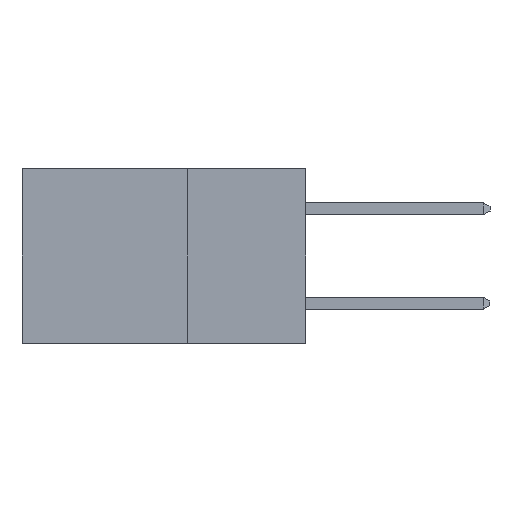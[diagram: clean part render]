
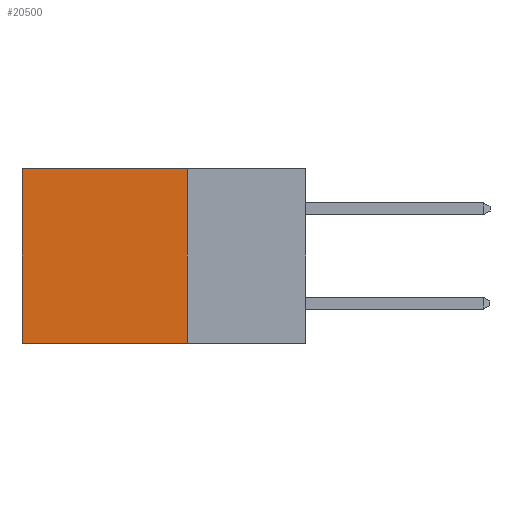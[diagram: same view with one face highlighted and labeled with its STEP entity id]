
A CAD part, left-side view. The second image highlights one B-rep face of the part: STEP entity #20500.
In plain terms, the highlighted planar face has unit normal (-1, 0, 0).
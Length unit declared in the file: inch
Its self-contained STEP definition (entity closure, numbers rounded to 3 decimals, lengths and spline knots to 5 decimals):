
#553 = FACE_OUTER_BOUND ( 'NONE', #14517, .T. ) ;
#619 = DIRECTION ( 'NONE',  ( 0., 0., -1. ) ) ;
#724 = VERTEX_POINT ( 'NONE', #21676 ) ;
#782 = CARTESIAN_POINT ( 'NONE',  ( 0.298, 0.6, 0. ) ) ;
#848 = PLANE ( 'NONE',  #11613 ) ;
#854 = ORIENTED_EDGE ( 'NONE', *, *, #21178, .F. ) ;
#1084 = CARTESIAN_POINT ( 'NONE',  ( 0.298, 0.25, 0. ) ) ;
#1229 = CARTESIAN_POINT ( 'NONE',  ( 0.298, 0.25, 0. ) ) ;
#1475 = LINE ( 'NONE', #15895, #19737 ) ;
#1815 = VERTEX_POINT ( 'NONE', #14395 ) ;
#2635 = DIRECTION ( 'NONE',  ( 0., 0., -1. ) ) ;
#3260 = ORIENTED_EDGE ( 'NONE', *, *, #22896, .T. ) ;
#3874 = LINE ( 'NONE', #1084, #17453 ) ;
#4594 = VERTEX_POINT ( 'NONE', #1229 ) ;
#4924 = ORIENTED_EDGE ( 'NONE', *, *, #20806, .T. ) ;
#6102 = CARTESIAN_POINT ( 'NONE',  ( 0.298, 0.25, 0. ) ) ;
#9103 = VECTOR ( 'NONE', #619, 39.37008 ) ;
#9323 = VERTEX_POINT ( 'NONE', #22578 ) ;
#9467 = CARTESIAN_POINT ( 'NONE',  ( 0.298, 0.25, 0. ) ) ;
#9681 = LINE ( 'NONE', #9467, #9103 ) ;
#11015 = LINE ( 'NONE', #782, #15130 ) ;
#11392 = DIRECTION ( 'NONE',  ( 0., 0., -1. ) ) ;
#11613 = AXIS2_PLACEMENT_3D ( 'NONE', #6102, #13232, #2635 ) ;
#11621 = DIRECTION ( 'NONE',  ( 0., 1., 0. ) ) ;
#12949 = ORIENTED_EDGE ( 'NONE', *, *, #18917, .F. ) ;
#13232 = DIRECTION ( 'NONE',  ( 1., 0., 0. ) ) ;
#14210 = DIRECTION ( 'NONE',  ( 0., 1., 0. ) ) ;
#14395 = CARTESIAN_POINT ( 'NONE',  ( 0.298, 0.6, 0. ) ) ;
#14517 = EDGE_LOOP ( 'NONE', ( #3260, #12949, #854, #4924 ) ) ;
#15130 = VECTOR ( 'NONE', #11392, 39.37008 ) ;
#15895 = CARTESIAN_POINT ( 'NONE',  ( 0.298, 0.25, -0.37 ) ) ;
#17453 = VECTOR ( 'NONE', #11621, 39.37008 ) ;
#18917 = EDGE_CURVE ( 'NONE', #9323, #724, #1475, .T. ) ;
#19737 = VECTOR ( 'NONE', #14210, 39.37008 ) ;
#20500 = ADVANCED_FACE ( 'NONE', ( #553 ), #848, .F. ) ;
#20806 = EDGE_CURVE ( 'NONE', #4594, #1815, #3874, .T. ) ;
#21178 = EDGE_CURVE ( 'NONE', #4594, #9323, #9681, .T. ) ;
#21676 = CARTESIAN_POINT ( 'NONE',  ( 0.298, 0.6, -0.37 ) ) ;
#22578 = CARTESIAN_POINT ( 'NONE',  ( 0.298, 0.25, -0.37 ) ) ;
#22896 = EDGE_CURVE ( 'NONE', #1815, #724, #11015, .T. ) ;
